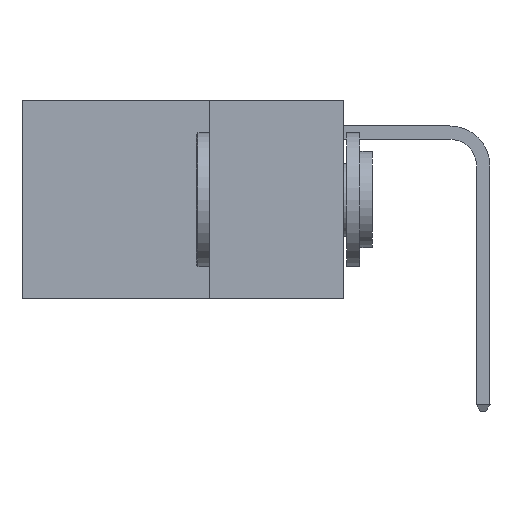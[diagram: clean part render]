
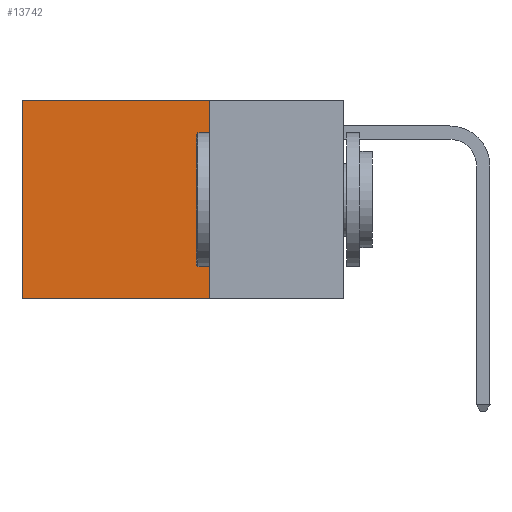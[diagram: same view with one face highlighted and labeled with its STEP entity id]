
A CAD part, left-side view. The second image highlights one B-rep face of the part: STEP entity #13742.
In plain terms, the highlighted planar face has unit normal (-1, 0, 0).
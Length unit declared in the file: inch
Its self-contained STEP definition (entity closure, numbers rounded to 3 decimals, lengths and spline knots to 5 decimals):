
#52 = FACE_OUTER_BOUND ( 'NONE', #22247, .T. ) ;
#1829 = CARTESIAN_POINT ( 'NONE',  ( 0.2625, 0.25, 0. ) ) ;
#2848 = VERTEX_POINT ( 'NONE', #18926 ) ;
#3690 = CARTESIAN_POINT ( 'NONE',  ( 0.2625, 0.25, 0. ) ) ;
#3843 = LINE ( 'NONE', #3690, #19119 ) ;
#3851 = ORIENTED_EDGE ( 'NONE', *, *, #8666, .F. ) ;
#3973 = DIRECTION ( 'NONE',  ( 0., 0., -1. ) ) ;
#4351 = PLANE ( 'NONE',  #11061 ) ;
#5083 = VECTOR ( 'NONE', #5970, 39.37008 ) ;
#5526 = VERTEX_POINT ( 'NONE', #17338 ) ;
#5826 = CARTESIAN_POINT ( 'NONE',  ( 0.2625, 0.6, 0. ) ) ;
#5970 = DIRECTION ( 'NONE',  ( 0., 1., 0. ) ) ;
#6291 = CARTESIAN_POINT ( 'NONE',  ( 0.2625, 0.25, 0. ) ) ;
#6749 = ORIENTED_EDGE ( 'NONE', *, *, #9262, .F. ) ;
#7622 = CARTESIAN_POINT ( 'NONE',  ( 0.2625, 0.6, -0.37 ) ) ;
#8216 = DIRECTION ( 'NONE',  ( 1., 0., 0. ) ) ;
#8339 = ORIENTED_EDGE ( 'NONE', *, *, #12907, .T. ) ;
#8666 = EDGE_CURVE ( 'NONE', #5526, #19474, #15303, .T. ) ;
#9231 = EDGE_CURVE ( 'NONE', #14802, #2848, #3843, .T. ) ;
#9262 = EDGE_CURVE ( 'NONE', #14802, #5526, #17342, .T. ) ;
#11061 = AXIS2_PLACEMENT_3D ( 'NONE', #6291, #8216, #21613 ) ;
#12907 = EDGE_CURVE ( 'NONE', #2848, #19474, #18697, .T. ) ;
#13661 = VECTOR ( 'NONE', #3973, 39.37008 ) ;
#13742 = ADVANCED_FACE ( 'NONE', ( #52 ), #4351, .F. ) ;
#14802 = VERTEX_POINT ( 'NONE', #18714 ) ;
#15207 = DIRECTION ( 'NONE',  ( 0., 1., 0. ) ) ;
#15303 = LINE ( 'NONE', #15555, #5083 ) ;
#15555 = CARTESIAN_POINT ( 'NONE',  ( 0.2625, 0.25, -0.37 ) ) ;
#16099 = DIRECTION ( 'NONE',  ( 0., 0., -1. ) ) ;
#17338 = CARTESIAN_POINT ( 'NONE',  ( 0.2625, 0.25, -0.37 ) ) ;
#17342 = LINE ( 'NONE', #1829, #21820 ) ;
#18697 = LINE ( 'NONE', #5826, #13661 ) ;
#18714 = CARTESIAN_POINT ( 'NONE',  ( 0.2625, 0.25, 0. ) ) ;
#18926 = CARTESIAN_POINT ( 'NONE',  ( 0.2625, 0.6, 0. ) ) ;
#19119 = VECTOR ( 'NONE', #15207, 39.37008 ) ;
#19474 = VERTEX_POINT ( 'NONE', #7622 ) ;
#21613 = DIRECTION ( 'NONE',  ( 0., 0., -1. ) ) ;
#21820 = VECTOR ( 'NONE', #16099, 39.37008 ) ;
#22247 = EDGE_LOOP ( 'NONE', ( #8339, #3851, #6749, #23174 ) ) ;
#23174 = ORIENTED_EDGE ( 'NONE', *, *, #9231, .T. ) ;
